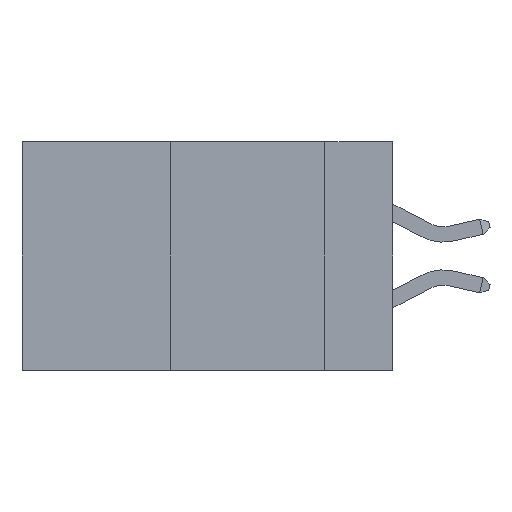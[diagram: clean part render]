
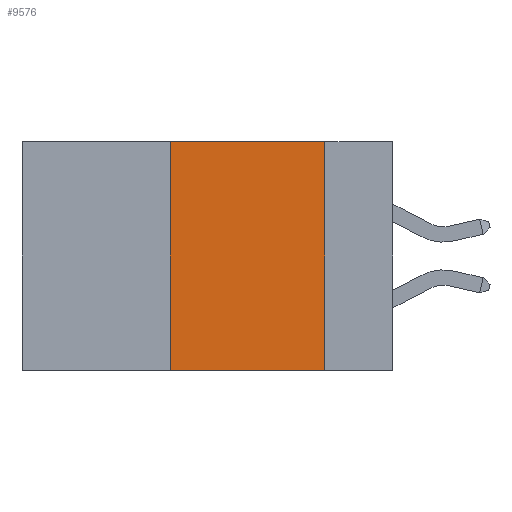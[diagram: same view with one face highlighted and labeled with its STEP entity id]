
A CAD part, left-side view. The second image highlights one B-rep face of the part: STEP entity #9576.
In plain terms, the highlighted planar face has unit normal (-1, 0, 0).
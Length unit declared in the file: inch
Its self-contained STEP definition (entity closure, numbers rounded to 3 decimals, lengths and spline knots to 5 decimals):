
#106 = EDGE_CURVE ( 'NONE', #6228, #4208, #6139, .T. ) ;
#195 = VECTOR ( 'NONE', #4425, 39.37008 ) ;
#213 = EDGE_CURVE ( 'NONE', #7087, #6506, #1375, .T. ) ;
#1375 = LINE ( 'NONE', #9072, #7323 ) ;
#1530 = CARTESIAN_POINT ( 'NONE',  ( 0., 0.11, 0. ) ) ;
#1593 = ORIENTED_EDGE ( 'NONE', *, *, #106, .F. ) ;
#1650 = ORIENTED_EDGE ( 'NONE', *, *, #3026, .F. ) ;
#2274 = CARTESIAN_POINT ( 'NONE',  ( 0., 0.11, -0.37 ) ) ;
#2290 = CARTESIAN_POINT ( 'NONE',  ( 0., 0.6, 0. ) ) ;
#2651 = LINE ( 'NONE', #8302, #6493 ) ;
#2778 = ORIENTED_EDGE ( 'NONE', *, *, #6314, .F. ) ;
#2834 = LINE ( 'NONE', #2958, #195 ) ;
#2958 = CARTESIAN_POINT ( 'NONE',  ( 0., 0.36, 0. ) ) ;
#3026 = EDGE_CURVE ( 'NONE', #4208, #6506, #2651, .T. ) ;
#3183 = ORIENTED_EDGE ( 'NONE', *, *, #213, .T. ) ;
#3764 = CARTESIAN_POINT ( 'NONE',  ( 0., 0.36, 0. ) ) ;
#4098 = VECTOR ( 'NONE', #6232, 39.37008 ) ;
#4208 = VERTEX_POINT ( 'NONE', #1530 ) ;
#4312 = EDGE_LOOP ( 'NONE', ( #1650, #1593, #2778, #3183 ) ) ;
#4380 = PLANE ( 'NONE',  #9078 ) ;
#4425 = DIRECTION ( 'NONE',  ( 0., 0., 1. ) ) ;
#4786 = DIRECTION ( 'NONE',  ( 0., -1., 0. ) ) ;
#5176 = DIRECTION ( 'NONE',  ( 0., 0., -1. ) ) ;
#5669 = CARTESIAN_POINT ( 'NONE',  ( 0., 0.36, -0.37 ) ) ;
#6139 = LINE ( 'NONE', #2290, #4098 ) ;
#6228 = VERTEX_POINT ( 'NONE', #3764 ) ;
#6232 = DIRECTION ( 'NONE',  ( 0., -1., 0. ) ) ;
#6314 = EDGE_CURVE ( 'NONE', #7087, #6228, #2834, .T. ) ;
#6493 = VECTOR ( 'NONE', #8335, 39.37008 ) ;
#6506 = VERTEX_POINT ( 'NONE', #2274 ) ;
#7087 = VERTEX_POINT ( 'NONE', #5669 ) ;
#7323 = VECTOR ( 'NONE', #4786, 39.37008 ) ;
#7859 = FACE_OUTER_BOUND ( 'NONE', #4312, .T. ) ;
#8024 = CARTESIAN_POINT ( 'NONE',  ( 0., 0.6, 0. ) ) ;
#8302 = CARTESIAN_POINT ( 'NONE',  ( 0., 0.11, 0. ) ) ;
#8335 = DIRECTION ( 'NONE',  ( 0., 0., -1. ) ) ;
#9072 = CARTESIAN_POINT ( 'NONE',  ( 0., 0.6, -0.37 ) ) ;
#9078 = AXIS2_PLACEMENT_3D ( 'NONE', #8024, #9385, #5176 ) ;
#9385 = DIRECTION ( 'NONE',  ( 1., 0., 0. ) ) ;
#9576 = ADVANCED_FACE ( 'NONE', ( #7859 ), #4380, .F. ) ;
